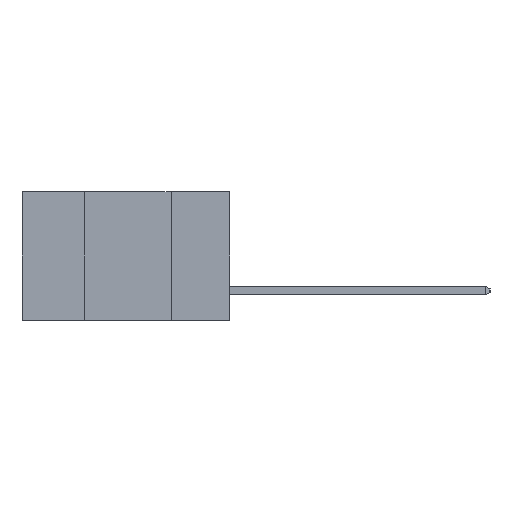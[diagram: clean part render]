
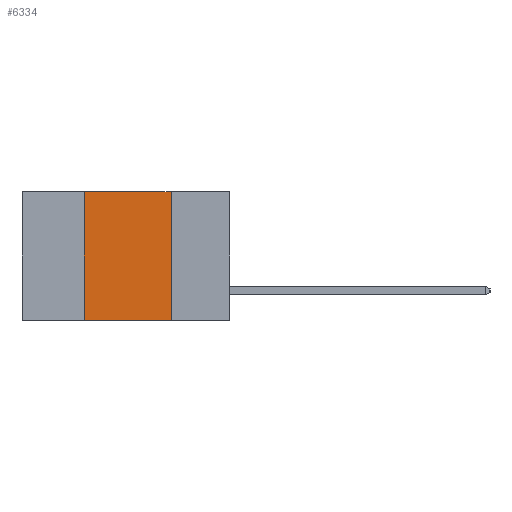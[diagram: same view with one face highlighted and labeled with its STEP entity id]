
A CAD part, left-side view. The second image highlights one B-rep face of the part: STEP entity #6334.
In plain terms, the highlighted planar face has unit normal (-1, 0, 0).
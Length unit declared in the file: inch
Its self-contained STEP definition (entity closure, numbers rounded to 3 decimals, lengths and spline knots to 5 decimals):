
#508 = VECTOR ( 'NONE', #9665, 39.37008 ) ;
#1916 = EDGE_CURVE ( 'NONE', #8996, #6027, #3375, .T. ) ;
#2128 = DIRECTION ( 'NONE',  ( 1., 0., 0. ) ) ;
#2307 = VERTEX_POINT ( 'NONE', #6154 ) ;
#3375 = LINE ( 'NONE', #8426, #508 ) ;
#3763 = CARTESIAN_POINT ( 'NONE',  ( 0., 0.42, 0. ) ) ;
#4478 = VECTOR ( 'NONE', #12323, 39.37008 ) ;
#5081 = VERTEX_POINT ( 'NONE', #8288 ) ;
#5453 = LINE ( 'NONE', #10664, #10620 ) ;
#5632 = ORIENTED_EDGE ( 'NONE', *, *, #9170, .F. ) ;
#6027 = VERTEX_POINT ( 'NONE', #3763 ) ;
#6154 = CARTESIAN_POINT ( 'NONE',  ( 0., 0.17, 0. ) ) ;
#6334 = ADVANCED_FACE ( 'NONE', ( #12810 ), #13473, .F. ) ;
#6982 = AXIS2_PLACEMENT_3D ( 'NONE', #8345, #2128, #9386 ) ;
#7220 = LINE ( 'NONE', #9216, #4478 ) ;
#8174 = ORIENTED_EDGE ( 'NONE', *, *, #12159, .F. ) ;
#8288 = CARTESIAN_POINT ( 'NONE',  ( 0., 0.17, -0.37 ) ) ;
#8345 = CARTESIAN_POINT ( 'NONE',  ( 0., 0.6, 0. ) ) ;
#8360 = EDGE_LOOP ( 'NONE', ( #8174, #5632, #13173, #13493 ) ) ;
#8426 = CARTESIAN_POINT ( 'NONE',  ( 0., 0.42, 0. ) ) ;
#8441 = EDGE_CURVE ( 'NONE', #8996, #5081, #5453, .T. ) ;
#8996 = VERTEX_POINT ( 'NONE', #12501 ) ;
#9170 = EDGE_CURVE ( 'NONE', #6027, #2307, #7220, .T. ) ;
#9216 = CARTESIAN_POINT ( 'NONE',  ( 0., 0.6, 0. ) ) ;
#9386 = DIRECTION ( 'NONE',  ( 0., 0., -1. ) ) ;
#9665 = DIRECTION ( 'NONE',  ( 0., 0., 1. ) ) ;
#10620 = VECTOR ( 'NONE', #11678, 39.37008 ) ;
#10664 = CARTESIAN_POINT ( 'NONE',  ( 0., 0.6, -0.37 ) ) ;
#11433 = VECTOR ( 'NONE', #12539, 39.37008 ) ;
#11520 = CARTESIAN_POINT ( 'NONE',  ( 0., 0.17, 0. ) ) ;
#11678 = DIRECTION ( 'NONE',  ( 0., -1., 0. ) ) ;
#11756 = LINE ( 'NONE', #11520, #11433 ) ;
#12159 = EDGE_CURVE ( 'NONE', #2307, #5081, #11756, .T. ) ;
#12323 = DIRECTION ( 'NONE',  ( 0., -1., 0. ) ) ;
#12501 = CARTESIAN_POINT ( 'NONE',  ( 0., 0.42, -0.37 ) ) ;
#12539 = DIRECTION ( 'NONE',  ( 0., 0., -1. ) ) ;
#12810 = FACE_OUTER_BOUND ( 'NONE', #8360, .T. ) ;
#13173 = ORIENTED_EDGE ( 'NONE', *, *, #1916, .F. ) ;
#13473 = PLANE ( 'NONE',  #6982 ) ;
#13493 = ORIENTED_EDGE ( 'NONE', *, *, #8441, .T. ) ;
